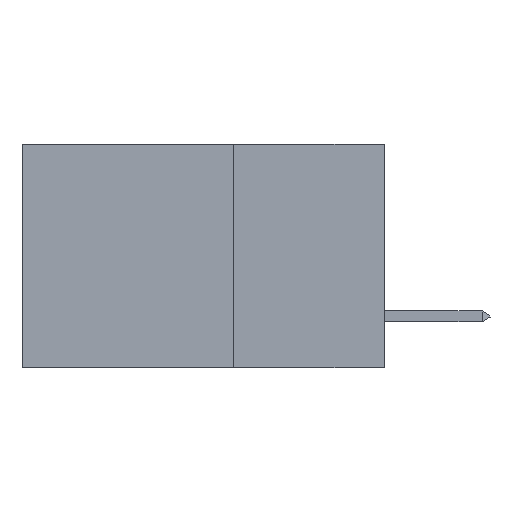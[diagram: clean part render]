
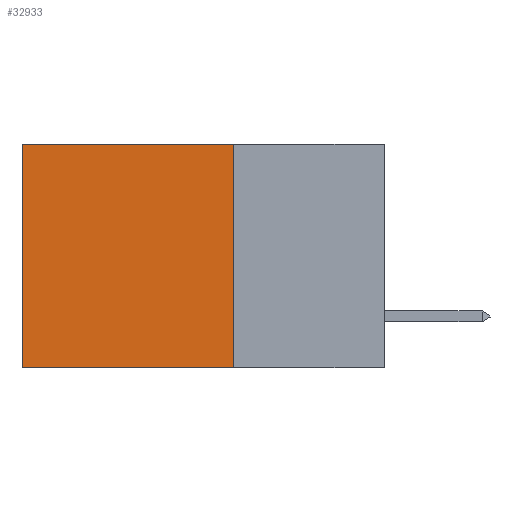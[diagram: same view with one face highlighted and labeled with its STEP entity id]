
A CAD part, left-side view. The second image highlights one B-rep face of the part: STEP entity #32933.
In plain terms, the highlighted planar face has unit normal (-1, 0, 0).
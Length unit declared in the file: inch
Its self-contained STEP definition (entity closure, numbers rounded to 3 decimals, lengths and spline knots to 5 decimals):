
#2849 = VECTOR ( 'NONE', #12291, 39.37008 ) ;
#3719 = LINE ( 'NONE', #23420, #2849 ) ;
#3728 = VERTEX_POINT ( 'NONE', #14081 ) ;
#3877 = VECTOR ( 'NONE', #3926, 39.37008 ) ;
#3926 = DIRECTION ( 'NONE',  ( 0., 1., 0. ) ) ;
#3932 = DIRECTION ( 'NONE',  ( 0., 0., -1. ) ) ;
#4991 = LINE ( 'NONE', #26034, #23257 ) ;
#7804 = EDGE_LOOP ( 'NONE', ( #19863, #30439, #12096, #29911 ) ) ;
#7841 = DIRECTION ( 'NONE',  ( 1., 0., 0. ) ) ;
#9557 = CARTESIAN_POINT ( 'NONE',  ( 0.2875, 0.25, 0. ) ) ;
#10273 = DIRECTION ( 'NONE',  ( 0., 0., -1. ) ) ;
#12096 = ORIENTED_EDGE ( 'NONE', *, *, #14752, .F. ) ;
#12291 = DIRECTION ( 'NONE',  ( 0., 1., 0. ) ) ;
#12949 = CARTESIAN_POINT ( 'NONE',  ( 0.2875, 0.25, 0. ) ) ;
#14081 = CARTESIAN_POINT ( 'NONE',  ( 0.2875, 0.25, -0.37 ) ) ;
#14648 = LINE ( 'NONE', #12949, #23730 ) ;
#14752 = EDGE_CURVE ( 'NONE', #18604, #3728, #14648, .T. ) ;
#16361 = AXIS2_PLACEMENT_3D ( 'NONE', #32697, #7841, #30146 ) ;
#17170 = CARTESIAN_POINT ( 'NONE',  ( 0.2875, 0.25, 0. ) ) ;
#18138 = VERTEX_POINT ( 'NONE', #25893 ) ;
#18604 = VERTEX_POINT ( 'NONE', #17170 ) ;
#18711 = EDGE_CURVE ( 'NONE', #3728, #30444, #3719, .T. ) ;
#19413 = EDGE_CURVE ( 'NONE', #18138, #30444, #4991, .T. ) ;
#19863 = ORIENTED_EDGE ( 'NONE', *, *, #19413, .T. ) ;
#21389 = CARTESIAN_POINT ( 'NONE',  ( 0.2875, 0.6, -0.37 ) ) ;
#23257 = VECTOR ( 'NONE', #3932, 39.37008 ) ;
#23420 = CARTESIAN_POINT ( 'NONE',  ( 0.2875, 0.25, -0.37 ) ) ;
#23730 = VECTOR ( 'NONE', #10273, 39.37008 ) ;
#24382 = FACE_OUTER_BOUND ( 'NONE', #7804, .T. ) ;
#25893 = CARTESIAN_POINT ( 'NONE',  ( 0.2875, 0.6, 0. ) ) ;
#26034 = CARTESIAN_POINT ( 'NONE',  ( 0.2875, 0.6, 0. ) ) ;
#27098 = PLANE ( 'NONE',  #16361 ) ;
#29911 = ORIENTED_EDGE ( 'NONE', *, *, #34409, .T. ) ;
#30146 = DIRECTION ( 'NONE',  ( 0., 0., -1. ) ) ;
#30439 = ORIENTED_EDGE ( 'NONE', *, *, #18711, .F. ) ;
#30444 = VERTEX_POINT ( 'NONE', #21389 ) ;
#31700 = LINE ( 'NONE', #9557, #3877 ) ;
#32697 = CARTESIAN_POINT ( 'NONE',  ( 0.2875, 0.25, 0. ) ) ;
#32933 = ADVANCED_FACE ( 'NONE', ( #24382 ), #27098, .F. ) ;
#34409 = EDGE_CURVE ( 'NONE', #18604, #18138, #31700, .T. ) ;
